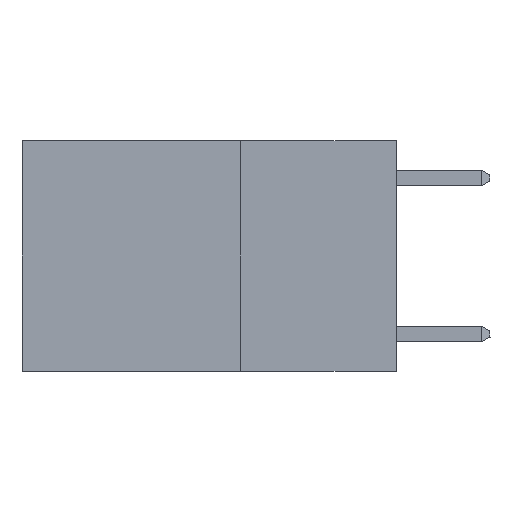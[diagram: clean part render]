
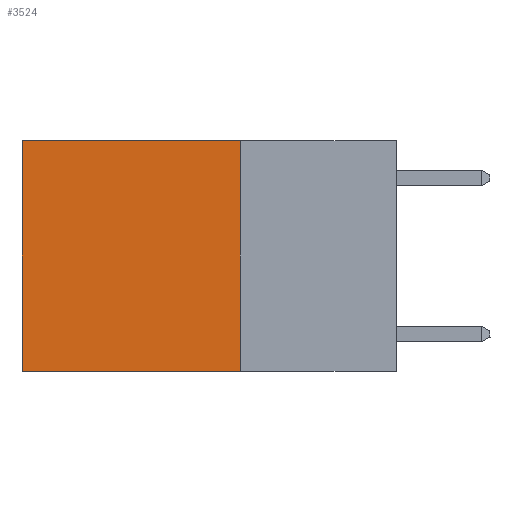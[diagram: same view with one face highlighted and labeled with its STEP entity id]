
A CAD part, left-side view. The second image highlights one B-rep face of the part: STEP entity #3524.
In plain terms, the highlighted planar face has unit normal (-1, 0, 0).
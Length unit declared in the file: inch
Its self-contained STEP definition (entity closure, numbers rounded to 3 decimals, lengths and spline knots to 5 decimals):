
#170 = DIRECTION ( 'NONE',  ( 1., 0., 0. ) ) ;
#349 = DIRECTION ( 'NONE',  ( 0., 0., -1. ) ) ;
#352 = VERTEX_POINT ( 'NONE', #3047 ) ;
#870 = LINE ( 'NONE', #12861, #16748 ) ;
#1125 = CARTESIAN_POINT ( 'NONE',  ( 0.2625, 0.25, -0.37 ) ) ;
#1154 = VECTOR ( 'NONE', #4679, 39.37008 ) ;
#3038 = CARTESIAN_POINT ( 'NONE',  ( 0.2625, 0.25, 0. ) ) ;
#3047 = CARTESIAN_POINT ( 'NONE',  ( 0.2625, 0.6, -0.37 ) ) ;
#3105 = CARTESIAN_POINT ( 'NONE',  ( 0.2625, 0.6, 0. ) ) ;
#3524 = ADVANCED_FACE ( 'NONE', ( #18816 ), #15583, .F. ) ;
#3961 = ORIENTED_EDGE ( 'NONE', *, *, #11623, .T. ) ;
#4608 = DIRECTION ( 'NONE',  ( 0., 1., 0. ) ) ;
#4679 = DIRECTION ( 'NONE',  ( 0., 0., -1. ) ) ;
#5840 = VECTOR ( 'NONE', #4608, 39.37008 ) ;
#6381 = ORIENTED_EDGE ( 'NONE', *, *, #13493, .F. ) ;
#7081 = VECTOR ( 'NONE', #349, 39.37008 ) ;
#7118 = EDGE_LOOP ( 'NONE', ( #14328, #6381, #18995, #3961 ) ) ;
#8176 = DIRECTION ( 'NONE',  ( 0., 1., 0. ) ) ;
#9406 = LINE ( 'NONE', #3105, #1154 ) ;
#9509 = CARTESIAN_POINT ( 'NONE',  ( 0.2625, 0.25, 0. ) ) ;
#9688 = CARTESIAN_POINT ( 'NONE',  ( 0.2625, 0.6, 0. ) ) ;
#10593 = VERTEX_POINT ( 'NONE', #14548 ) ;
#11062 = DIRECTION ( 'NONE',  ( 0., 0., -1. ) ) ;
#11623 = EDGE_CURVE ( 'NONE', #10593, #11894, #13970, .T. ) ;
#11672 = EDGE_CURVE ( 'NONE', #11894, #352, #9406, .T. ) ;
#11894 = VERTEX_POINT ( 'NONE', #9688 ) ;
#12861 = CARTESIAN_POINT ( 'NONE',  ( 0.2625, 0.25, -0.37 ) ) ;
#13493 = EDGE_CURVE ( 'NONE', #14341, #352, #870, .T. ) ;
#13970 = LINE ( 'NONE', #3038, #5840 ) ;
#14328 = ORIENTED_EDGE ( 'NONE', *, *, #11672, .T. ) ;
#14341 = VERTEX_POINT ( 'NONE', #1125 ) ;
#14548 = CARTESIAN_POINT ( 'NONE',  ( 0.2625, 0.25, 0. ) ) ;
#15583 = PLANE ( 'NONE',  #15689 ) ;
#15689 = AXIS2_PLACEMENT_3D ( 'NONE', #9509, #170, #11062 ) ;
#16748 = VECTOR ( 'NONE', #8176, 39.37008 ) ;
#17624 = EDGE_CURVE ( 'NONE', #10593, #14341, #18656, .T. ) ;
#18656 = LINE ( 'NONE', #18768, #7081 ) ;
#18768 = CARTESIAN_POINT ( 'NONE',  ( 0.2625, 0.25, 0. ) ) ;
#18816 = FACE_OUTER_BOUND ( 'NONE', #7118, .T. ) ;
#18995 = ORIENTED_EDGE ( 'NONE', *, *, #17624, .F. ) ;
